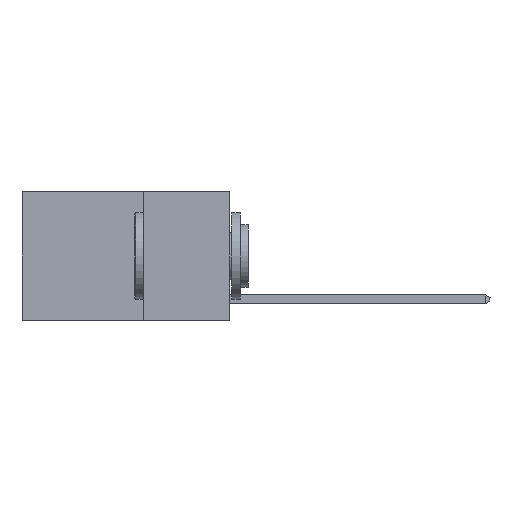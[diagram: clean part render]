
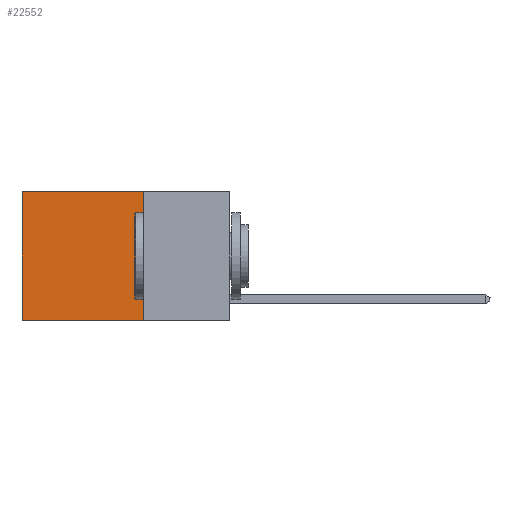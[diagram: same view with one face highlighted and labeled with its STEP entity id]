
A CAD part, left-side view. The second image highlights one B-rep face of the part: STEP entity #22552.
In plain terms, the highlighted planar face has unit normal (-1, 0, 0).
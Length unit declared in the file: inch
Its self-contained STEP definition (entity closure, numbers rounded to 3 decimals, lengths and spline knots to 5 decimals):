
#40 = CARTESIAN_POINT ( 'NONE',  ( 0.2625, 0.6, -0.37 ) ) ;
#1095 = DIRECTION ( 'NONE',  ( 0., 1., 0. ) ) ;
#1663 = VECTOR ( 'NONE', #2987, 39.37008 ) ;
#2987 = DIRECTION ( 'NONE',  ( 0., 0., -1. ) ) ;
#3611 = VECTOR ( 'NONE', #1095, 39.37008 ) ;
#4134 = CARTESIAN_POINT ( 'NONE',  ( 0.2625, 0.25, 0. ) ) ;
#4197 = ORIENTED_EDGE ( 'NONE', *, *, #16168, .T. ) ;
#4210 = CARTESIAN_POINT ( 'NONE',  ( 0.2625, 0.25, 0. ) ) ;
#6116 = VERTEX_POINT ( 'NONE', #6770 ) ;
#6543 = DIRECTION ( 'NONE',  ( 0., 0., -1. ) ) ;
#6770 = CARTESIAN_POINT ( 'NONE',  ( 0.2625, 0.25, -0.37 ) ) ;
#7131 = EDGE_CURVE ( 'NONE', #6116, #21233, #14900, .T. ) ;
#8268 = FACE_OUTER_BOUND ( 'NONE', #20845, .T. ) ;
#8601 = LINE ( 'NONE', #22507, #1663 ) ;
#12151 = DIRECTION ( 'NONE',  ( 1., 0., 0. ) ) ;
#12463 = LINE ( 'NONE', #14168, #15283 ) ;
#13151 = ORIENTED_EDGE ( 'NONE', *, *, #23140, .F. ) ;
#13168 = LINE ( 'NONE', #18652, #19550 ) ;
#13312 = AXIS2_PLACEMENT_3D ( 'NONE', #4210, #12151, #6543 ) ;
#13418 = VERTEX_POINT ( 'NONE', #4134 ) ;
#14168 = CARTESIAN_POINT ( 'NONE',  ( 0.2625, 0.6, 0. ) ) ;
#14505 = ORIENTED_EDGE ( 'NONE', *, *, #22609, .T. ) ;
#14900 = LINE ( 'NONE', #15037, #3611 ) ;
#15037 = CARTESIAN_POINT ( 'NONE',  ( 0.2625, 0.25, -0.37 ) ) ;
#15283 = VECTOR ( 'NONE', #22099, 39.37008 ) ;
#16168 = EDGE_CURVE ( 'NONE', #17675, #21233, #12463, .T. ) ;
#16438 = PLANE ( 'NONE',  #13312 ) ;
#17675 = VERTEX_POINT ( 'NONE', #22003 ) ;
#18652 = CARTESIAN_POINT ( 'NONE',  ( 0.2625, 0.25, 0. ) ) ;
#19550 = VECTOR ( 'NONE', #21112, 39.37008 ) ;
#20845 = EDGE_LOOP ( 'NONE', ( #4197, #21355, #13151, #14505 ) ) ;
#21112 = DIRECTION ( 'NONE',  ( 0., 1., 0. ) ) ;
#21233 = VERTEX_POINT ( 'NONE', #40 ) ;
#21355 = ORIENTED_EDGE ( 'NONE', *, *, #7131, .F. ) ;
#22003 = CARTESIAN_POINT ( 'NONE',  ( 0.2625, 0.6, 0. ) ) ;
#22099 = DIRECTION ( 'NONE',  ( 0., 0., -1. ) ) ;
#22507 = CARTESIAN_POINT ( 'NONE',  ( 0.2625, 0.25, 0. ) ) ;
#22552 = ADVANCED_FACE ( 'NONE', ( #8268 ), #16438, .F. ) ;
#22609 = EDGE_CURVE ( 'NONE', #13418, #17675, #13168, .T. ) ;
#23140 = EDGE_CURVE ( 'NONE', #13418, #6116, #8601, .T. ) ;
